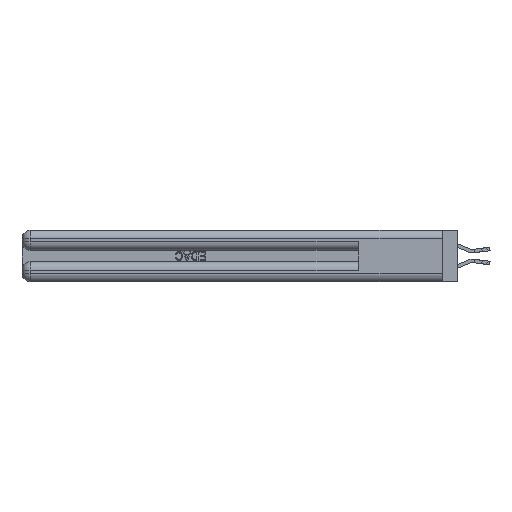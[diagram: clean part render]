
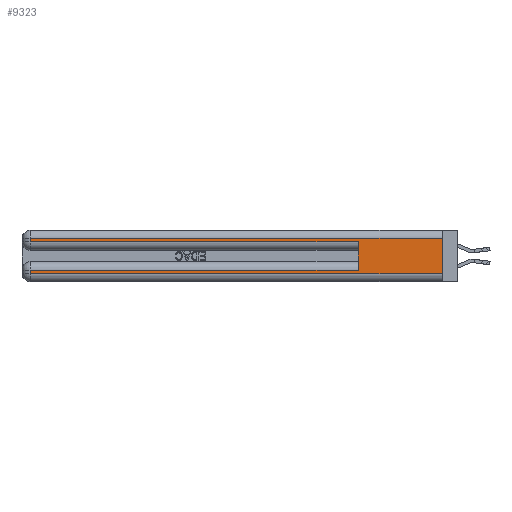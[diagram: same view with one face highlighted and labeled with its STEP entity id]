
A CAD part, left-side view. The second image highlights one B-rep face of the part: STEP entity #9323.
In plain terms, the highlighted planar face has unit normal (-1, 0, 0).
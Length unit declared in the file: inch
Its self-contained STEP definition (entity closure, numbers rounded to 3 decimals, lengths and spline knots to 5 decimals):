
#663 = ORIENTED_EDGE ( 'NONE', *, *, #12846, .T. ) ;
#940 = VECTOR ( 'NONE', #1424, 39.37008 ) ;
#1424 = DIRECTION ( 'NONE',  ( 0., 0., -1. ) ) ;
#1748 = DIRECTION ( 'NONE',  ( 0., 0., -1. ) ) ;
#1992 = VERTEX_POINT ( 'NONE', #33017 ) ;
#2065 = CARTESIAN_POINT ( 'NONE',  ( 0., 0., 0.085 ) ) ;
#4326 = EDGE_CURVE ( 'NONE', #29697, #10847, #37506, .T. ) ;
#4355 = CARTESIAN_POINT ( 'NONE',  ( 0., 0.6, 0.085 ) ) ;
#5050 = LINE ( 'NONE', #2065, #19088 ) ;
#5140 = DIRECTION ( 'NONE',  ( 0., 0., -1. ) ) ;
#5262 = CARTESIAN_POINT ( 'NONE',  ( 0., 0., 0.37 ) ) ;
#5291 = VERTEX_POINT ( 'NONE', #4355 ) ;
#5438 = VECTOR ( 'NONE', #23840, 39.37008 ) ;
#6032 = VECTOR ( 'NONE', #5140, 39.37008 ) ;
#7733 = LINE ( 'NONE', #28973, #14985 ) ;
#8036 = VECTOR ( 'NONE', #28070, 39.37008 ) ;
#9188 = EDGE_LOOP ( 'NONE', ( #31941, #32084, #10315, #33556, #11676, #663, #22646, #28191 ) ) ;
#9323 = ADVANCED_FACE ( 'NONE', ( #13575 ), #11155, .F. ) ;
#9532 = EDGE_CURVE ( 'NONE', #15408, #26227, #30922, .T. ) ;
#10069 = LINE ( 'NONE', #10433, #940 ) ;
#10315 = ORIENTED_EDGE ( 'NONE', *, *, #17177, .T. ) ;
#10433 = CARTESIAN_POINT ( 'NONE',  ( 0., 2.94, 0.37 ) ) ;
#10847 = VERTEX_POINT ( 'NONE', #20028 ) ;
#11155 = PLANE ( 'NONE',  #16496 ) ;
#11676 = ORIENTED_EDGE ( 'NONE', *, *, #24018, .F. ) ;
#11737 = CARTESIAN_POINT ( 'NONE',  ( 0., 0., 0.31 ) ) ;
#12846 = EDGE_CURVE ( 'NONE', #5291, #15408, #5050, .T. ) ;
#12914 = EDGE_CURVE ( 'NONE', #29697, #27058, #22456, .T. ) ;
#13575 = FACE_OUTER_BOUND ( 'NONE', #9188, .T. ) ;
#13666 = LINE ( 'NONE', #35958, #5438 ) ;
#14035 = CARTESIAN_POINT ( 'NONE',  ( 0., 2.94, 0.085 ) ) ;
#14920 = DIRECTION ( 'NONE',  ( 0., -1., 0. ) ) ;
#14985 = VECTOR ( 'NONE', #32183, 39.37008 ) ;
#15408 = VERTEX_POINT ( 'NONE', #14035 ) ;
#15454 = VECTOR ( 'NONE', #16400, 39.37008 ) ;
#16400 = DIRECTION ( 'NONE',  ( 0., 0., -1. ) ) ;
#16496 = AXIS2_PLACEMENT_3D ( 'NONE', #23179, #35949, #1748 ) ;
#17177 = EDGE_CURVE ( 'NONE', #10847, #1992, #10069, .T. ) ;
#17823 = DIRECTION ( 'NONE',  ( 0., 1., 0. ) ) ;
#18605 = CARTESIAN_POINT ( 'NONE',  ( 0., 2.94, 0.37 ) ) ;
#19088 = VECTOR ( 'NONE', #17823, 39.37008 ) ;
#20028 = CARTESIAN_POINT ( 'NONE',  ( 0., 2.94, 0.31 ) ) ;
#22456 = LINE ( 'NONE', #5262, #6032 ) ;
#22646 = ORIENTED_EDGE ( 'NONE', *, *, #9532, .T. ) ;
#23092 = CARTESIAN_POINT ( 'NONE',  ( 0., 0., 0.285 ) ) ;
#23179 = CARTESIAN_POINT ( 'NONE',  ( 0., 0., 0.37 ) ) ;
#23588 = CARTESIAN_POINT ( 'NONE',  ( 0., 0., 0.31 ) ) ;
#23840 = DIRECTION ( 'NONE',  ( 0., 0., 1. ) ) ;
#24018 = EDGE_CURVE ( 'NONE', #5291, #24783, #13666, .T. ) ;
#24783 = VERTEX_POINT ( 'NONE', #38914 ) ;
#26227 = VERTEX_POINT ( 'NONE', #34000 ) ;
#27058 = VERTEX_POINT ( 'NONE', #38264 ) ;
#28070 = DIRECTION ( 'NONE',  ( 0., 1., 0. ) ) ;
#28191 = ORIENTED_EDGE ( 'NONE', *, *, #32477, .T. ) ;
#28973 = CARTESIAN_POINT ( 'NONE',  ( 0., 0., 0.06 ) ) ;
#29697 = VERTEX_POINT ( 'NONE', #23588 ) ;
#30922 = LINE ( 'NONE', #18605, #15454 ) ;
#31941 = ORIENTED_EDGE ( 'NONE', *, *, #12914, .F. ) ;
#32084 = ORIENTED_EDGE ( 'NONE', *, *, #4326, .T. ) ;
#32183 = DIRECTION ( 'NONE',  ( 0., -1., 0. ) ) ;
#32477 = EDGE_CURVE ( 'NONE', #26227, #27058, #7733, .T. ) ;
#33017 = CARTESIAN_POINT ( 'NONE',  ( 0., 2.94, 0.285 ) ) ;
#33556 = ORIENTED_EDGE ( 'NONE', *, *, #34829, .T. ) ;
#34000 = CARTESIAN_POINT ( 'NONE',  ( 0., 2.94, 0.06 ) ) ;
#34613 = VECTOR ( 'NONE', #14920, 39.37008 ) ;
#34829 = EDGE_CURVE ( 'NONE', #1992, #24783, #39899, .T. ) ;
#35949 = DIRECTION ( 'NONE',  ( 1., 0., 0. ) ) ;
#35958 = CARTESIAN_POINT ( 'NONE',  ( 0., 0.6, 0.145 ) ) ;
#37506 = LINE ( 'NONE', #11737, #8036 ) ;
#38264 = CARTESIAN_POINT ( 'NONE',  ( 0., 0., 0.06 ) ) ;
#38914 = CARTESIAN_POINT ( 'NONE',  ( 0., 0.6, 0.285 ) ) ;
#39899 = LINE ( 'NONE', #23092, #34613 ) ;
